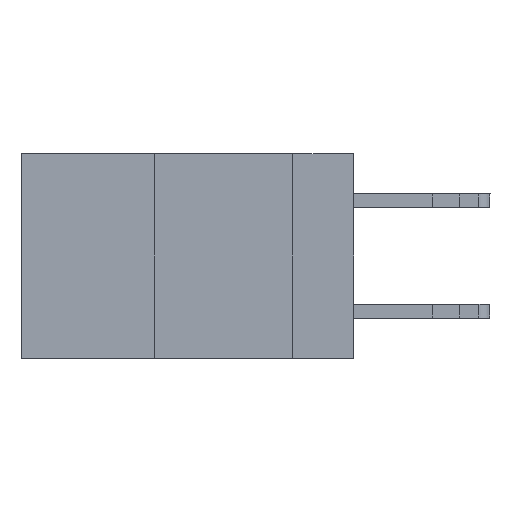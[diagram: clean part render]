
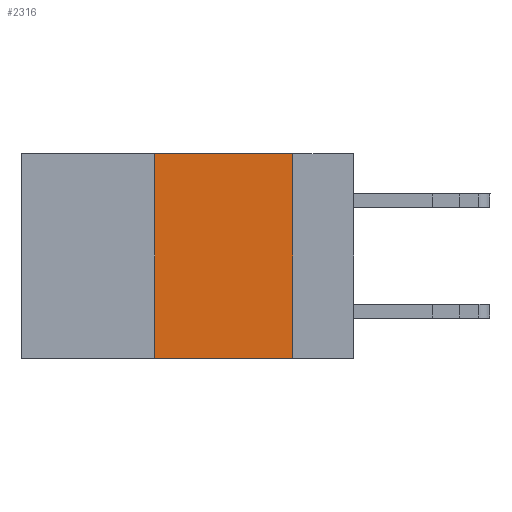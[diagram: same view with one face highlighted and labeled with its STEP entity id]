
A CAD part, left-side view. The second image highlights one B-rep face of the part: STEP entity #2316.
In plain terms, the highlighted planar face has unit normal (-1, 0, 0).
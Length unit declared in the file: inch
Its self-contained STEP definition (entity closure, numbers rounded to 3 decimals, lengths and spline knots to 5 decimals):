
#107 = CARTESIAN_POINT ( 'NONE',  ( 0., 0.36, 0. ) ) ;
#326 = LINE ( 'NONE', #25468, #24187 ) ;
#1714 = CARTESIAN_POINT ( 'NONE',  ( 0., 0.36, 0. ) ) ;
#2267 = VERTEX_POINT ( 'NONE', #107 ) ;
#2316 = ADVANCED_FACE ( 'NONE', ( #4295 ), #26449, .F. ) ;
#3686 = DIRECTION ( 'NONE',  ( 0., -1., 0. ) ) ;
#4295 = FACE_OUTER_BOUND ( 'NONE', #7519, .T. ) ;
#4489 = VECTOR ( 'NONE', #28980, 39.37008 ) ;
#6143 = EDGE_CURVE ( 'NONE', #14147, #19833, #13359, .T. ) ;
#7519 = EDGE_LOOP ( 'NONE', ( #10138, #14288, #17075, #15651 ) ) ;
#9866 = EDGE_CURVE ( 'NONE', #2267, #20713, #10589, .T. ) ;
#10138 = ORIENTED_EDGE ( 'NONE', *, *, #20005, .F. ) ;
#10589 = LINE ( 'NONE', #22041, #4489 ) ;
#11800 = DIRECTION ( 'NONE',  ( 0., 0., -1. ) ) ;
#13300 = DIRECTION ( 'NONE',  ( 1., 0., 0. ) ) ;
#13359 = LINE ( 'NONE', #15570, #28093 ) ;
#14147 = VERTEX_POINT ( 'NONE', #18998 ) ;
#14288 = ORIENTED_EDGE ( 'NONE', *, *, #9866, .F. ) ;
#15570 = CARTESIAN_POINT ( 'NONE',  ( 0., 0.6, -0.37 ) ) ;
#15651 = ORIENTED_EDGE ( 'NONE', *, *, #6143, .T. ) ;
#17075 = ORIENTED_EDGE ( 'NONE', *, *, #20684, .F. ) ;
#17617 = CARTESIAN_POINT ( 'NONE',  ( 0., 0.11, -0.37 ) ) ;
#18998 = CARTESIAN_POINT ( 'NONE',  ( 0., 0.36, -0.37 ) ) ;
#19822 = LINE ( 'NONE', #1714, #23064 ) ;
#19833 = VERTEX_POINT ( 'NONE', #17617 ) ;
#19881 = AXIS2_PLACEMENT_3D ( 'NONE', #24010, #13300, #11800 ) ;
#20005 = EDGE_CURVE ( 'NONE', #20713, #19833, #326, .T. ) ;
#20201 = CARTESIAN_POINT ( 'NONE',  ( 0., 0.11, 0. ) ) ;
#20684 = EDGE_CURVE ( 'NONE', #14147, #2267, #19822, .T. ) ;
#20713 = VERTEX_POINT ( 'NONE', #20201 ) ;
#20723 = DIRECTION ( 'NONE',  ( 0., 0., -1. ) ) ;
#22041 = CARTESIAN_POINT ( 'NONE',  ( 0., 0.6, 0. ) ) ;
#22829 = DIRECTION ( 'NONE',  ( 0., 0., 1. ) ) ;
#23064 = VECTOR ( 'NONE', #22829, 39.37008 ) ;
#24010 = CARTESIAN_POINT ( 'NONE',  ( 0., 0.6, 0. ) ) ;
#24187 = VECTOR ( 'NONE', #20723, 39.37008 ) ;
#25468 = CARTESIAN_POINT ( 'NONE',  ( 0., 0.11, 0. ) ) ;
#26449 = PLANE ( 'NONE',  #19881 ) ;
#28093 = VECTOR ( 'NONE', #3686, 39.37008 ) ;
#28980 = DIRECTION ( 'NONE',  ( 0., -1., 0. ) ) ;
